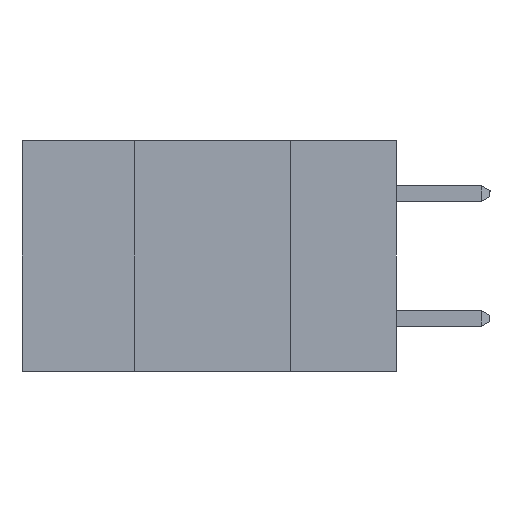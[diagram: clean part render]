
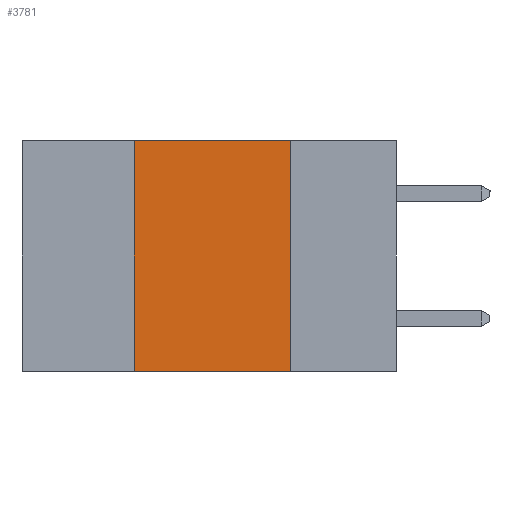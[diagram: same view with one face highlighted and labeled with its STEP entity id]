
A CAD part, left-side view. The second image highlights one B-rep face of the part: STEP entity #3781.
In plain terms, the highlighted planar face has unit normal (-1, 0, 0).
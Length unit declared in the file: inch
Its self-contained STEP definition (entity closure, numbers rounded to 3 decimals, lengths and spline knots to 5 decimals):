
#185 = DIRECTION ( 'NONE',  ( 1., 0., 0. ) ) ;
#208 = CARTESIAN_POINT ( 'NONE',  ( 0., 0.42, -0.37 ) ) ;
#416 = CARTESIAN_POINT ( 'NONE',  ( 0., 0.17, 0. ) ) ;
#1387 = LINE ( 'NONE', #5007, #3196 ) ;
#1409 = EDGE_CURVE ( 'NONE', #2073, #1706, #4551, .T. ) ;
#1421 = VERTEX_POINT ( 'NONE', #7134 ) ;
#1545 = EDGE_CURVE ( 'NONE', #1421, #7722, #11931, .T. ) ;
#1706 = VERTEX_POINT ( 'NONE', #9551 ) ;
#2073 = VERTEX_POINT ( 'NONE', #416 ) ;
#2294 = ORIENTED_EDGE ( 'NONE', *, *, #1545, .F. ) ;
#2932 = EDGE_LOOP ( 'NONE', ( #7568, #3453, #2294, #7154 ) ) ;
#3196 = VECTOR ( 'NONE', #4829, 39.37008 ) ;
#3453 = ORIENTED_EDGE ( 'NONE', *, *, #6074, .F. ) ;
#3581 = DIRECTION ( 'NONE',  ( 0., 0., -1. ) ) ;
#3641 = DIRECTION ( 'NONE',  ( 0., 0., 1. ) ) ;
#3781 = ADVANCED_FACE ( 'NONE', ( #8446 ), #5421, .F. ) ;
#4551 = LINE ( 'NONE', #11630, #9439 ) ;
#4829 = DIRECTION ( 'NONE',  ( 0., -1., 0. ) ) ;
#4950 = CARTESIAN_POINT ( 'NONE',  ( 0., 0.42, 0. ) ) ;
#5007 = CARTESIAN_POINT ( 'NONE',  ( 0., 0.6, -0.37 ) ) ;
#5421 = PLANE ( 'NONE',  #7872 ) ;
#6074 = EDGE_CURVE ( 'NONE', #7722, #2073, #7966, .T. ) ;
#6992 = DIRECTION ( 'NONE',  ( 0., -1., 0. ) ) ;
#7134 = CARTESIAN_POINT ( 'NONE',  ( 0., 0.42, -0.37 ) ) ;
#7154 = ORIENTED_EDGE ( 'NONE', *, *, #10434, .T. ) ;
#7568 = ORIENTED_EDGE ( 'NONE', *, *, #1409, .F. ) ;
#7722 = VERTEX_POINT ( 'NONE', #4950 ) ;
#7872 = AXIS2_PLACEMENT_3D ( 'NONE', #11046, #185, #8382 ) ;
#7966 = LINE ( 'NONE', #9613, #11830 ) ;
#8297 = VECTOR ( 'NONE', #3641, 39.37008 ) ;
#8382 = DIRECTION ( 'NONE',  ( 0., 0., -1. ) ) ;
#8446 = FACE_OUTER_BOUND ( 'NONE', #2932, .T. ) ;
#9439 = VECTOR ( 'NONE', #3581, 39.37008 ) ;
#9551 = CARTESIAN_POINT ( 'NONE',  ( 0., 0.17, -0.37 ) ) ;
#9613 = CARTESIAN_POINT ( 'NONE',  ( 0., 0.6, 0. ) ) ;
#10434 = EDGE_CURVE ( 'NONE', #1421, #1706, #1387, .T. ) ;
#11046 = CARTESIAN_POINT ( 'NONE',  ( 0., 0.6, 0. ) ) ;
#11630 = CARTESIAN_POINT ( 'NONE',  ( 0., 0.17, -0.37 ) ) ;
#11830 = VECTOR ( 'NONE', #6992, 39.37008 ) ;
#11931 = LINE ( 'NONE', #208, #8297 ) ;
